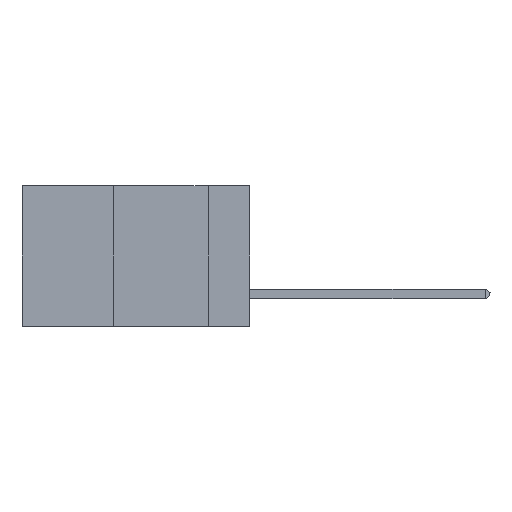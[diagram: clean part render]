
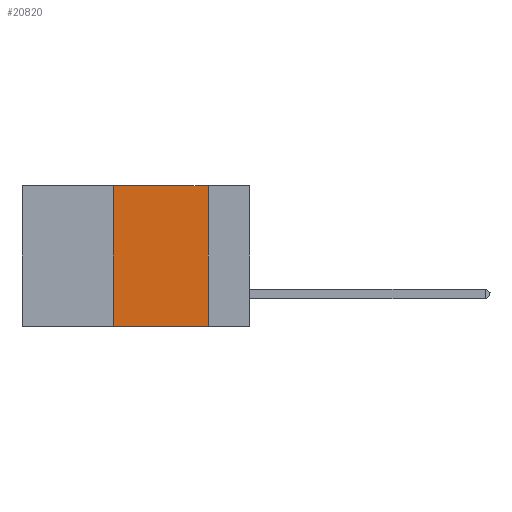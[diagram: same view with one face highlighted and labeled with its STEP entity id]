
A CAD part, left-side view. The second image highlights one B-rep face of the part: STEP entity #20820.
In plain terms, the highlighted planar face has unit normal (-1, 0, 0).
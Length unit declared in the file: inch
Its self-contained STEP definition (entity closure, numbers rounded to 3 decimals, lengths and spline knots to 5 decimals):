
#563 = ORIENTED_EDGE ( 'NONE', *, *, #652, .F. ) ;
#652 = EDGE_CURVE ( 'NONE', #33502, #33536, #31702, .T. ) ;
#693 = DIRECTION ( 'NONE',  ( 0., 0., 1. ) ) ;
#2265 = PLANE ( 'NONE',  #3298 ) ;
#3298 = AXIS2_PLACEMENT_3D ( 'NONE', #30524, #15454, #22835 ) ;
#9044 = EDGE_LOOP ( 'NONE', ( #563, #21080, #26879, #15906 ) ) ;
#9412 = VECTOR ( 'NONE', #14910, 39.37008 ) ;
#10742 = DIRECTION ( 'NONE',  ( 0., 0., -1. ) ) ;
#10844 = LINE ( 'NONE', #12972, #30735 ) ;
#12972 = CARTESIAN_POINT ( 'NONE',  ( 0., 0.6, 0. ) ) ;
#13078 = DIRECTION ( 'NONE',  ( 0., -1., 0. ) ) ;
#13717 = CARTESIAN_POINT ( 'NONE',  ( 0., 0.11, 0. ) ) ;
#14910 = DIRECTION ( 'NONE',  ( 0., -1., 0. ) ) ;
#15454 = DIRECTION ( 'NONE',  ( 1., 0., 0. ) ) ;
#15906 = ORIENTED_EDGE ( 'NONE', *, *, #25131, .T. ) ;
#16120 = EDGE_CURVE ( 'NONE', #23484, #33502, #10844, .T. ) ;
#16609 = FACE_OUTER_BOUND ( 'NONE', #9044, .T. ) ;
#19141 = CARTESIAN_POINT ( 'NONE',  ( 0., 0.11, -0.37 ) ) ;
#20820 = ADVANCED_FACE ( 'NONE', ( #16609 ), #2265, .F. ) ;
#21080 = ORIENTED_EDGE ( 'NONE', *, *, #16120, .F. ) ;
#21698 = CARTESIAN_POINT ( 'NONE',  ( 0., 0.36, 0. ) ) ;
#22626 = CARTESIAN_POINT ( 'NONE',  ( 0., 0.6, -0.37 ) ) ;
#22835 = DIRECTION ( 'NONE',  ( 0., 0., -1. ) ) ;
#23484 = VERTEX_POINT ( 'NONE', #32106 ) ;
#25131 = EDGE_CURVE ( 'NONE', #33485, #33536, #25260, .T. ) ;
#25260 = LINE ( 'NONE', #22626, #9412 ) ;
#26879 = ORIENTED_EDGE ( 'NONE', *, *, #29423, .F. ) ;
#28644 = CARTESIAN_POINT ( 'NONE',  ( 0., 0.11, 0. ) ) ;
#29190 = LINE ( 'NONE', #21698, #31984 ) ;
#29423 = EDGE_CURVE ( 'NONE', #33485, #23484, #29190, .T. ) ;
#29699 = VECTOR ( 'NONE', #10742, 39.37008 ) ;
#30524 = CARTESIAN_POINT ( 'NONE',  ( 0., 0.6, 0. ) ) ;
#30735 = VECTOR ( 'NONE', #13078, 39.37008 ) ;
#31629 = CARTESIAN_POINT ( 'NONE',  ( 0., 0.36, -0.37 ) ) ;
#31702 = LINE ( 'NONE', #28644, #29699 ) ;
#31984 = VECTOR ( 'NONE', #693, 39.37008 ) ;
#32106 = CARTESIAN_POINT ( 'NONE',  ( 0., 0.36, 0. ) ) ;
#33485 = VERTEX_POINT ( 'NONE', #31629 ) ;
#33502 = VERTEX_POINT ( 'NONE', #13717 ) ;
#33536 = VERTEX_POINT ( 'NONE', #19141 ) ;
